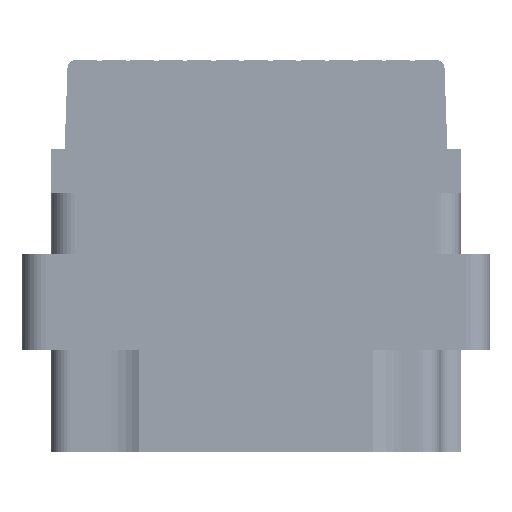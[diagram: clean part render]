
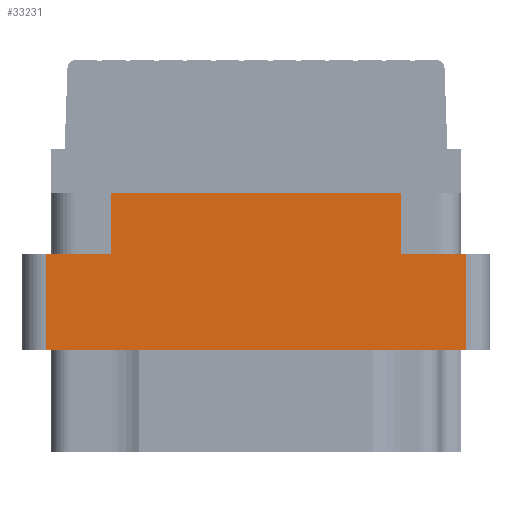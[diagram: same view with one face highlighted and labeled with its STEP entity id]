
A CAD part, left-side view. The second image highlights one B-rep face of the part: STEP entity #33231.
In plain terms, the highlighted planar face has unit normal (-1, 0, 0).
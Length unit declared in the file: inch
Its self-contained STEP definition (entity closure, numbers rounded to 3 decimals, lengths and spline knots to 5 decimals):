
#3635 = DIRECTION ( 'NONE',  ( 0., 0., 1. ) ) ;
#4598 = ORIENTED_EDGE ( 'NONE', *, *, #62788, .T. ) ;
#6004 = VERTEX_POINT ( 'NONE', #39440 ) ;
#6247 = VECTOR ( 'NONE', #32275, 39.37008 ) ;
#6725 = LINE ( 'NONE', #18149, #34656 ) ;
#7502 = VECTOR ( 'NONE', #43185, 39.37008 ) ;
#8232 = VERTEX_POINT ( 'NONE', #52511 ) ;
#9453 = CARTESIAN_POINT ( 'NONE',  ( -1.359, -0.3825, -0.117 ) ) ;
#9706 = ORIENTED_EDGE ( 'NONE', *, *, #36150, .F. ) ;
#10113 = PLANE ( 'NONE',  #31947 ) ;
#12949 = CARTESIAN_POINT ( 'NONE',  ( -1.359, -0.3825, -0.277 ) ) ;
#13015 = VECTOR ( 'NONE', #36132, 39.37008 ) ;
#14376 = CARTESIAN_POINT ( 'NONE',  ( -1.359, 0.3825, -0.277 ) ) ;
#14827 = CARTESIAN_POINT ( 'NONE',  ( -1.359, 0., -0.277 ) ) ;
#16596 = VECTOR ( 'NONE', #62482, 39.37008 ) ;
#16874 = DIRECTION ( 'NONE',  ( 0., -1., 0. ) ) ;
#18149 = CARTESIAN_POINT ( 'NONE',  ( -1.359, 0., -0.529 ) ) ;
#18529 = LINE ( 'NONE', #40278, #16596 ) ;
#21123 = CARTESIAN_POINT ( 'NONE',  ( -1.359, 0.555, -0.277 ) ) ;
#21456 = DIRECTION ( 'NONE',  ( 0., 0., 1. ) ) ;
#22238 = CARTESIAN_POINT ( 'NONE',  ( -1.359, 0.617, -0.117 ) ) ;
#24264 = EDGE_CURVE ( 'NONE', #55713, #8232, #48369, .T. ) ;
#24378 = LINE ( 'NONE', #14376, #13015 ) ;
#26415 = CARTESIAN_POINT ( 'NONE',  ( -1.359, 0., -0.277 ) ) ;
#26539 = VECTOR ( 'NONE', #3635, 39.37008 ) ;
#26775 = EDGE_CURVE ( 'NONE', #49550, #52850, #18529, .T. ) ;
#28491 = DIRECTION ( 'NONE',  ( 0., 1., 0. ) ) ;
#31641 = EDGE_LOOP ( 'NONE', ( #54457, #62446, #9706, #67940, #70389, #4598, #68946, #45936 ) ) ;
#31862 = DIRECTION ( 'NONE',  ( -1., 0., 0. ) ) ;
#31947 = AXIS2_PLACEMENT_3D ( 'NONE', #52622, #31862, #41874 ) ;
#32105 = CARTESIAN_POINT ( 'NONE',  ( -1.359, -0.555, -0.529 ) ) ;
#32154 = LINE ( 'NONE', #43236, #49377 ) ;
#32275 = DIRECTION ( 'NONE',  ( 0., -1., 0. ) ) ;
#33231 = ADVANCED_FACE ( 'NONE', ( #46535 ), #10113, .T. ) ;
#34656 = VECTOR ( 'NONE', #28491, 39.37008 ) ;
#36132 = DIRECTION ( 'NONE',  ( 0., 0., 1. ) ) ;
#36150 = EDGE_CURVE ( 'NONE', #38889, #52850, #6725, .T. ) ;
#38889 = VERTEX_POINT ( 'NONE', #32105 ) ;
#39440 = CARTESIAN_POINT ( 'NONE',  ( -1.359, 0.3825, -0.277 ) ) ;
#39720 = VERTEX_POINT ( 'NONE', #69069 ) ;
#40278 = CARTESIAN_POINT ( 'NONE',  ( -1.359, 0.555, -0.798 ) ) ;
#41874 = DIRECTION ( 'NONE',  ( 0., 0., 1. ) ) ;
#43185 = DIRECTION ( 'NONE',  ( 0., -1., 0. ) ) ;
#43236 = CARTESIAN_POINT ( 'NONE',  ( -1.359, -0.555, -0.798 ) ) ;
#45633 = VERTEX_POINT ( 'NONE', #9453 ) ;
#45936 = ORIENTED_EDGE ( 'NONE', *, *, #53768, .F. ) ;
#46535 = FACE_OUTER_BOUND ( 'NONE', #31641, .T. ) ;
#47486 = LINE ( 'NONE', #26415, #7502 ) ;
#48369 = LINE ( 'NONE', #14827, #6247 ) ;
#49377 = VECTOR ( 'NONE', #21456, 39.37008 ) ;
#49550 = VERTEX_POINT ( 'NONE', #21123 ) ;
#50983 = VECTOR ( 'NONE', #16874, 39.37008 ) ;
#52216 = LINE ( 'NONE', #12949, #26539 ) ;
#52405 = CARTESIAN_POINT ( 'NONE',  ( -1.359, 0.555, -0.529 ) ) ;
#52511 = CARTESIAN_POINT ( 'NONE',  ( -1.359, -0.555, -0.277 ) ) ;
#52622 = CARTESIAN_POINT ( 'NONE',  ( -1.359, -0.617, -0.798 ) ) ;
#52850 = VERTEX_POINT ( 'NONE', #52405 ) ;
#53768 = EDGE_CURVE ( 'NONE', #6004, #39720, #24378, .T. ) ;
#54457 = ORIENTED_EDGE ( 'NONE', *, *, #55600, .F. ) ;
#55600 = EDGE_CURVE ( 'NONE', #49550, #6004, #47486, .T. ) ;
#55713 = VERTEX_POINT ( 'NONE', #60371 ) ;
#60371 = CARTESIAN_POINT ( 'NONE',  ( -1.359, -0.3825, -0.277 ) ) ;
#62446 = ORIENTED_EDGE ( 'NONE', *, *, #26775, .T. ) ;
#62482 = DIRECTION ( 'NONE',  ( 0., 0., -1. ) ) ;
#62788 = EDGE_CURVE ( 'NONE', #55713, #45633, #52216, .T. ) ;
#62903 = EDGE_CURVE ( 'NONE', #38889, #8232, #32154, .T. ) ;
#65823 = LINE ( 'NONE', #22238, #50983 ) ;
#67940 = ORIENTED_EDGE ( 'NONE', *, *, #62903, .T. ) ;
#68510 = EDGE_CURVE ( 'NONE', #39720, #45633, #65823, .T. ) ;
#68946 = ORIENTED_EDGE ( 'NONE', *, *, #68510, .F. ) ;
#69069 = CARTESIAN_POINT ( 'NONE',  ( -1.359, 0.3825, -0.117 ) ) ;
#70389 = ORIENTED_EDGE ( 'NONE', *, *, #24264, .F. ) ;
